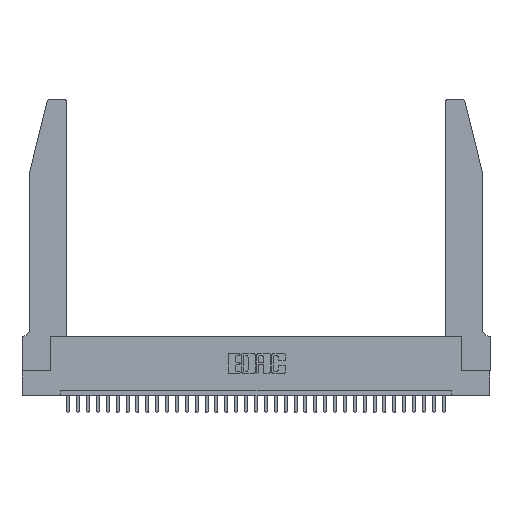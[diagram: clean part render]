
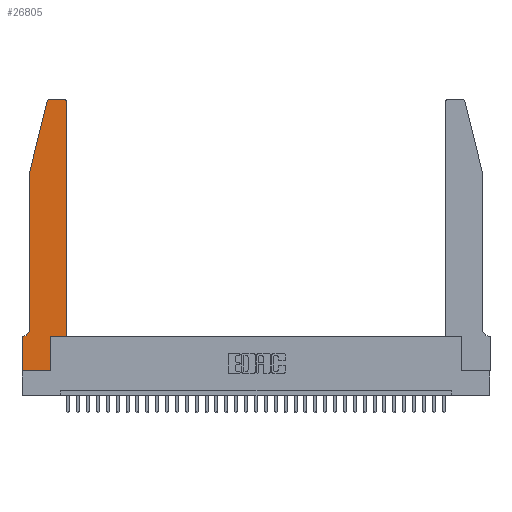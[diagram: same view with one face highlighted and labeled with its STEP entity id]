
A CAD part, top view. The second image highlights one B-rep face of the part: STEP entity #26805.
In plain terms, the highlighted planar face has unit normal (0, 0, 1).
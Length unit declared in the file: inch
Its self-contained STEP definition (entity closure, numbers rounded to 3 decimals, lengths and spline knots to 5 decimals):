
#262 = ORIENTED_EDGE ( 'NONE', *, *, #24753, .T. ) ;
#574 = EDGE_CURVE ( 'NONE', #27492, #8754, #14981, .T. ) ;
#1482 = VECTOR ( 'NONE', #27805, 39.37008 ) ;
#1811 = CIRCLE ( 'NONE', #3903, 0.03 ) ;
#2474 = ORIENTED_EDGE ( 'NONE', *, *, #32713, .T. ) ;
#2976 = CARTESIAN_POINT ( 'NONE',  ( 0., 0., 0.37 ) ) ;
#3144 = EDGE_CURVE ( 'NONE', #15008, #9639, #12686, .T. ) ;
#3692 = VECTOR ( 'NONE', #17733, 39.37008 ) ;
#3903 = AXIS2_PLACEMENT_3D ( 'NONE', #15670, #4958, #5301 ) ;
#4261 = EDGE_CURVE ( 'NONE', #32306, #33711, #28063, .T. ) ;
#4609 = DIRECTION ( 'NONE',  ( 0., 0., -1. ) ) ;
#4958 = DIRECTION ( 'NONE',  ( 0., 0., 1. ) ) ;
#5301 = DIRECTION ( 'NONE',  ( 1., 0., 0. ) ) ;
#5646 = CARTESIAN_POINT ( 'NONE',  ( 0.0055, 0.35, 0.37 ) ) ;
#5654 = DIRECTION ( 'NONE',  ( 0., 0., 1. ) ) ;
#5678 = DIRECTION ( 'NONE',  ( 0., -1., 0. ) ) ;
#6490 = AXIS2_PLACEMENT_3D ( 'NONE', #32313, #5654, #27019 ) ;
#6584 = ORIENTED_EDGE ( 'NONE', *, *, #23983, .T. ) ;
#7152 = VERTEX_POINT ( 'NONE', #12946 ) ;
#7456 = CARTESIAN_POINT ( 'NONE',  ( 0.2605, 2.75, 0.37 ) ) ;
#7578 = VERTEX_POINT ( 'NONE', #29003 ) ;
#7653 = CARTESIAN_POINT ( 'NONE',  ( 0.25487, 2.72718, 0.37 ) ) ;
#7801 = LINE ( 'NONE', #21978, #21143 ) ;
#8754 = VERTEX_POINT ( 'NONE', #30332 ) ;
#9264 = LINE ( 'NONE', #21678, #13018 ) ;
#9639 = VERTEX_POINT ( 'NONE', #32634 ) ;
#9881 = CARTESIAN_POINT ( 'NONE',  ( 0.0055, 0.42, 0.37 ) ) ;
#10236 = DIRECTION ( 'NONE',  ( 0., 0., 1. ) ) ;
#10937 = PLANE ( 'NONE',  #6490 ) ;
#11563 = ORIENTED_EDGE ( 'NONE', *, *, #23601, .T. ) ;
#11765 = VERTEX_POINT ( 'NONE', #7653 ) ;
#12097 = CIRCLE ( 'NONE', #26998, 0.03 ) ;
#12140 = ORIENTED_EDGE ( 'NONE', *, *, #17996, .T. ) ;
#12320 = CARTESIAN_POINT ( 'NONE',  ( 0.0755, 0.42, 0.37 ) ) ;
#12686 = LINE ( 'NONE', #12796, #13509 ) ;
#12796 = CARTESIAN_POINT ( 'NONE',  ( 0.2865, 0.35, 0.37 ) ) ;
#12946 = CARTESIAN_POINT ( 'NONE',  ( 0.0755, 2., 0.37 ) ) ;
#13018 = VECTOR ( 'NONE', #13555, 39.37008 ) ;
#13378 = CARTESIAN_POINT ( 'NONE',  ( 0.4505, 0.35, 0.37 ) ) ;
#13509 = VECTOR ( 'NONE', #15450, 39.37008 ) ;
#13555 = DIRECTION ( 'NONE',  ( -1., 0., 0. ) ) ;
#14981 = LINE ( 'NONE', #13378, #3692 ) ;
#15008 = VERTEX_POINT ( 'NONE', #30341 ) ;
#15450 = DIRECTION ( 'NONE',  ( 0., 1., 0. ) ) ;
#15670 = CARTESIAN_POINT ( 'NONE',  ( 0.284, 2.72, 0.37 ) ) ;
#16000 = FACE_OUTER_BOUND ( 'NONE', #28692, .T. ) ;
#16118 = EDGE_CURVE ( 'NONE', #24299, #7578, #23645, .T. ) ;
#16705 = ORIENTED_EDGE ( 'NONE', *, *, #4261, .T. ) ;
#17733 = DIRECTION ( 'NONE',  ( 0., 1., 0. ) ) ;
#17996 = EDGE_CURVE ( 'NONE', #33711, #11765, #1811, .T. ) ;
#17999 = CARTESIAN_POINT ( 'NONE',  ( 0.4205, 2.72, 0.37 ) ) ;
#18397 = EDGE_CURVE ( 'NONE', #11765, #7152, #34437, .T. ) ;
#19131 = CARTESIAN_POINT ( 'NONE',  ( 0.4505, 0.35, 0.37 ) ) ;
#19960 = CIRCLE ( 'NONE', #34049, 0.07 ) ;
#21100 = LINE ( 'NONE', #30257, #1482 ) ;
#21143 = VECTOR ( 'NONE', #5678, 39.37008 ) ;
#21617 = DIRECTION ( 'NONE',  ( 1., 0., 0. ) ) ;
#21621 = ORIENTED_EDGE ( 'NONE', *, *, #574, .T. ) ;
#21678 = CARTESIAN_POINT ( 'NONE',  ( 0.0755, 0.35, 0.37 ) ) ;
#21978 = CARTESIAN_POINT ( 'NONE',  ( 0.0755, 2., 0.37 ) ) ;
#22166 = DIRECTION ( 'NONE',  ( -0.239, -0.971, 0. ) ) ;
#22423 = CARTESIAN_POINT ( 'NONE',  ( 0.4205, 2.75, 0.37 ) ) ;
#22508 = EDGE_CURVE ( 'NONE', #27207, #24991, #19960, .T. ) ;
#23601 = EDGE_CURVE ( 'NONE', #9639, #27492, #21100, .T. ) ;
#23645 = LINE ( 'NONE', #24485, #34594 ) ;
#23983 = EDGE_CURVE ( 'NONE', #7152, #27207, #7801, .T. ) ;
#24299 = VERTEX_POINT ( 'NONE', #32687 ) ;
#24485 = CARTESIAN_POINT ( 'NONE',  ( 0., 0., 0.37 ) ) ;
#24753 = EDGE_CURVE ( 'NONE', #7578, #15008, #31162, .T. ) ;
#24991 = VERTEX_POINT ( 'NONE', #5646 ) ;
#25212 = CARTESIAN_POINT ( 'NONE',  ( 0.0755, 2., 0.37 ) ) ;
#25952 = DIRECTION ( 'NONE',  ( -1., 0., 0. ) ) ;
#26805 = ADVANCED_FACE ( 'NONE', ( #16000 ), #10937, .T. ) ;
#26998 = AXIS2_PLACEMENT_3D ( 'NONE', #17999, #10236, #28765 ) ;
#27019 = DIRECTION ( 'NONE',  ( 1., 0., 0. ) ) ;
#27207 = VERTEX_POINT ( 'NONE', #12320 ) ;
#27492 = VERTEX_POINT ( 'NONE', #19131 ) ;
#27805 = DIRECTION ( 'NONE',  ( 1., 0., 0. ) ) ;
#28063 = LINE ( 'NONE', #7456, #28912 ) ;
#28692 = EDGE_LOOP ( 'NONE', ( #16705, #12140, #34022, #6584, #33181, #2474, #33849, #262, #32515, #11563, #21621, #29964 ) ) ;
#28765 = DIRECTION ( 'NONE',  ( 1., 0., 0. ) ) ;
#28912 = VECTOR ( 'NONE', #33670, 39.37008 ) ;
#29003 = CARTESIAN_POINT ( 'NONE',  ( 0., 0., 0.37 ) ) ;
#29964 = ORIENTED_EDGE ( 'NONE', *, *, #33920, .T. ) ;
#30257 = CARTESIAN_POINT ( 'NONE',  ( 0.4505, 0.35, 0.37 ) ) ;
#30332 = CARTESIAN_POINT ( 'NONE',  ( 0.4505, 2.72, 0.37 ) ) ;
#30341 = CARTESIAN_POINT ( 'NONE',  ( 0.2865, 0., 0.37 ) ) ;
#30815 = CARTESIAN_POINT ( 'NONE',  ( 0.284, 2.75, 0.37 ) ) ;
#31162 = LINE ( 'NONE', #2976, #32388 ) ;
#32298 = DIRECTION ( 'NONE',  ( 0., -1., 0. ) ) ;
#32306 = VERTEX_POINT ( 'NONE', #22423 ) ;
#32313 = CARTESIAN_POINT ( 'NONE',  ( 0., 0.35, 0.37 ) ) ;
#32388 = VECTOR ( 'NONE', #21617, 39.37008 ) ;
#32515 = ORIENTED_EDGE ( 'NONE', *, *, #3144, .T. ) ;
#32634 = CARTESIAN_POINT ( 'NONE',  ( 0.2865, 0.35, 0.37 ) ) ;
#32687 = CARTESIAN_POINT ( 'NONE',  ( 0., 0.35, 0.37 ) ) ;
#32713 = EDGE_CURVE ( 'NONE', #24991, #24299, #9264, .T. ) ;
#32736 = VECTOR ( 'NONE', #22166, 39.37008 ) ;
#33181 = ORIENTED_EDGE ( 'NONE', *, *, #22508, .T. ) ;
#33670 = DIRECTION ( 'NONE',  ( -1., 0., 0. ) ) ;
#33711 = VERTEX_POINT ( 'NONE', #30815 ) ;
#33849 = ORIENTED_EDGE ( 'NONE', *, *, #16118, .T. ) ;
#33920 = EDGE_CURVE ( 'NONE', #8754, #32306, #12097, .T. ) ;
#34022 = ORIENTED_EDGE ( 'NONE', *, *, #18397, .T. ) ;
#34049 = AXIS2_PLACEMENT_3D ( 'NONE', #9881, #4609, #25952 ) ;
#34437 = LINE ( 'NONE', #25212, #32736 ) ;
#34594 = VECTOR ( 'NONE', #32298, 39.37008 ) ;
